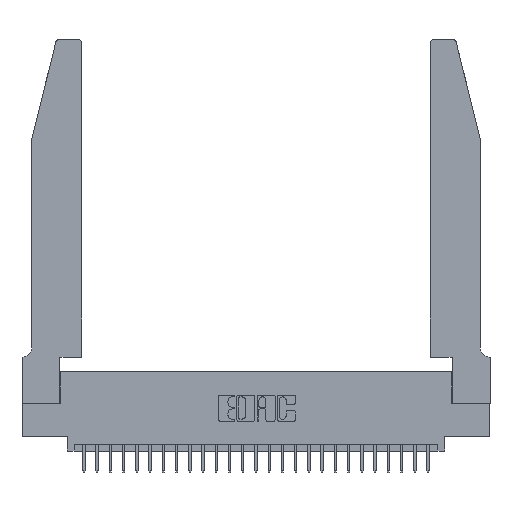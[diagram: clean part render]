
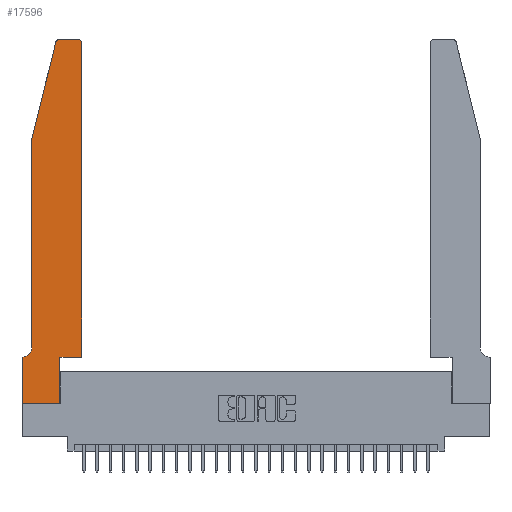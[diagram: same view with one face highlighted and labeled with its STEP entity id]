
A CAD part, top view. The second image highlights one B-rep face of the part: STEP entity #17596.
In plain terms, the highlighted planar face has unit normal (0, 0, 1).
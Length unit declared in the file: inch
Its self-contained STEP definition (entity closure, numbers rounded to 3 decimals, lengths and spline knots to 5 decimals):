
#159 = CARTESIAN_POINT ( 'NONE',  ( 0.284, 2.72, 0.37 ) ) ;
#443 = PLANE ( 'NONE',  #22139 ) ;
#631 = CARTESIAN_POINT ( 'NONE',  ( 0.2865, 0., 0.37 ) ) ;
#815 = DIRECTION ( 'NONE',  ( -1., 0., 0. ) ) ;
#893 = ORIENTED_EDGE ( 'NONE', *, *, #7026, .T. ) ;
#1359 = LINE ( 'NONE', #11806, #23803 ) ;
#1435 = VERTEX_POINT ( 'NONE', #25277 ) ;
#1686 = ORIENTED_EDGE ( 'NONE', *, *, #3947, .T. ) ;
#1898 = CIRCLE ( 'NONE', #14327, 0.07 ) ;
#2181 = DIRECTION ( 'NONE',  ( -1., 0., 0. ) ) ;
#2206 = CARTESIAN_POINT ( 'NONE',  ( 0.4505, 0.35, 0.37 ) ) ;
#2349 = CARTESIAN_POINT ( 'NONE',  ( 0.0755, 2., 0.37 ) ) ;
#2489 = DIRECTION ( 'NONE',  ( 1., 0., 0. ) ) ;
#3582 = CARTESIAN_POINT ( 'NONE',  ( 0., 0., 0.37 ) ) ;
#3947 = EDGE_CURVE ( 'NONE', #19488, #25809, #1359, .T. ) ;
#4549 = VECTOR ( 'NONE', #9200, 39.37008 ) ;
#4614 = DIRECTION ( 'NONE',  ( 0., -1., 0. ) ) ;
#4648 = EDGE_CURVE ( 'NONE', #10174, #25925, #24745, .T. ) ;
#4990 = DIRECTION ( 'NONE',  ( 0., 0., 1. ) ) ;
#5090 = DIRECTION ( 'NONE',  ( 0., 0., 1. ) ) ;
#5293 = ORIENTED_EDGE ( 'NONE', *, *, #12631, .T. ) ;
#5517 = AXIS2_PLACEMENT_3D ( 'NONE', #159, #15505, #2489 ) ;
#5609 = VERTEX_POINT ( 'NONE', #19052 ) ;
#6517 = ORIENTED_EDGE ( 'NONE', *, *, #21836, .T. ) ;
#7026 = EDGE_CURVE ( 'NONE', #5609, #13934, #12187, .T. ) ;
#7449 = VECTOR ( 'NONE', #4614, 39.37008 ) ;
#7740 = ORIENTED_EDGE ( 'NONE', *, *, #13269, .T. ) ;
#7753 = EDGE_CURVE ( 'NONE', #24947, #1435, #21922, .T. ) ;
#8119 = CARTESIAN_POINT ( 'NONE',  ( 0.2865, 0.35, 0.37 ) ) ;
#8923 = CARTESIAN_POINT ( 'NONE',  ( 0.0755, 2., 0.37 ) ) ;
#9200 = DIRECTION ( 'NONE',  ( 0., 1., 0. ) ) ;
#9277 = EDGE_CURVE ( 'NONE', #13934, #20509, #24633, .T. ) ;
#9488 = AXIS2_PLACEMENT_3D ( 'NONE', #18006, #5090, #20184 ) ;
#9513 = ORIENTED_EDGE ( 'NONE', *, *, #4648, .T. ) ;
#9641 = DIRECTION ( 'NONE',  ( 1., 0., 0. ) ) ;
#10174 = VERTEX_POINT ( 'NONE', #16843 ) ;
#11126 = VECTOR ( 'NONE', #9641, 39.37008 ) ;
#11675 = ORIENTED_EDGE ( 'NONE', *, *, #7753, .T. ) ;
#11806 = CARTESIAN_POINT ( 'NONE',  ( 0.2605, 2.75, 0.37 ) ) ;
#12187 = LINE ( 'NONE', #8923, #17905 ) ;
#12242 = CARTESIAN_POINT ( 'NONE',  ( 0., 0., 0.37 ) ) ;
#12516 = CARTESIAN_POINT ( 'NONE',  ( 0.4205, 2.75, 0.37 ) ) ;
#12631 = EDGE_CURVE ( 'NONE', #1435, #17283, #25854, .T. ) ;
#12876 = CIRCLE ( 'NONE', #5517, 0.03 ) ;
#13269 = EDGE_CURVE ( 'NONE', #26946, #24947, #21765, .T. ) ;
#13934 = VERTEX_POINT ( 'NONE', #25986 ) ;
#14024 = CARTESIAN_POINT ( 'NONE',  ( 0.0755, 0.35, 0.37 ) ) ;
#14327 = AXIS2_PLACEMENT_3D ( 'NONE', #28095, #15198, #2181 ) ;
#14463 = ORIENTED_EDGE ( 'NONE', *, *, #26116, .T. ) ;
#15198 = DIRECTION ( 'NONE',  ( 0., 0., -1. ) ) ;
#15223 = DIRECTION ( 'NONE',  ( 0., 1., 0. ) ) ;
#15376 = LINE ( 'NONE', #3582, #26164 ) ;
#15505 = DIRECTION ( 'NONE',  ( 0., 0., 1. ) ) ;
#15629 = FACE_OUTER_BOUND ( 'NONE', #18023, .T. ) ;
#15644 = EDGE_CURVE ( 'NONE', #25368, #10174, #16778, .T. ) ;
#16150 = DIRECTION ( 'NONE',  ( -1., 0., 0. ) ) ;
#16542 = DIRECTION ( 'NONE',  ( 1., 0., 0. ) ) ;
#16617 = CARTESIAN_POINT ( 'NONE',  ( 0., 0., 0.37 ) ) ;
#16778 = LINE ( 'NONE', #14024, #21154 ) ;
#16843 = CARTESIAN_POINT ( 'NONE',  ( 0., 0.35, 0.37 ) ) ;
#16967 = ORIENTED_EDGE ( 'NONE', *, *, #18683, .T. ) ;
#17283 = VERTEX_POINT ( 'NONE', #25377 ) ;
#17596 = ADVANCED_FACE ( 'NONE', ( #15629 ), #443, .T. ) ;
#17847 = ORIENTED_EDGE ( 'NONE', *, *, #26317, .T. ) ;
#17905 = VECTOR ( 'NONE', #23905, 39.37008 ) ;
#17909 = CARTESIAN_POINT ( 'NONE',  ( 0., 0.35, 0.37 ) ) ;
#18006 = CARTESIAN_POINT ( 'NONE',  ( 0.4205, 2.72, 0.37 ) ) ;
#18023 = EDGE_LOOP ( 'NONE', ( #1686, #16967, #893, #25917, #14463, #20744, #9513, #6517, #7740, #11675, #5293, #17847 ) ) ;
#18494 = CARTESIAN_POINT ( 'NONE',  ( 0.284, 2.75, 0.37 ) ) ;
#18683 = EDGE_CURVE ( 'NONE', #25809, #5609, #12876, .T. ) ;
#18850 = CARTESIAN_POINT ( 'NONE',  ( 0.0755, 0.42, 0.37 ) ) ;
#19009 = VECTOR ( 'NONE', #25138, 39.37008 ) ;
#19052 = CARTESIAN_POINT ( 'NONE',  ( 0.25487, 2.72718, 0.37 ) ) ;
#19488 = VERTEX_POINT ( 'NONE', #12516 ) ;
#19539 = CIRCLE ( 'NONE', #9488, 0.03 ) ;
#20086 = DIRECTION ( 'NONE',  ( 1., 0., 0. ) ) ;
#20184 = DIRECTION ( 'NONE',  ( 1., 0., 0. ) ) ;
#20509 = VERTEX_POINT ( 'NONE', #18850 ) ;
#20744 = ORIENTED_EDGE ( 'NONE', *, *, #15644, .T. ) ;
#21154 = VECTOR ( 'NONE', #815, 39.37008 ) ;
#21765 = LINE ( 'NONE', #24236, #4549 ) ;
#21836 = EDGE_CURVE ( 'NONE', #25925, #26946, #15376, .T. ) ;
#21922 = LINE ( 'NONE', #24687, #11126 ) ;
#22139 = AXIS2_PLACEMENT_3D ( 'NONE', #17909, #4990, #20086 ) ;
#23803 = VECTOR ( 'NONE', #16150, 39.37008 ) ;
#23905 = DIRECTION ( 'NONE',  ( -0.239, -0.971, 0. ) ) ;
#24236 = CARTESIAN_POINT ( 'NONE',  ( 0.2865, 0.35, 0.37 ) ) ;
#24633 = LINE ( 'NONE', #2349, #7449 ) ;
#24687 = CARTESIAN_POINT ( 'NONE',  ( 0.4505, 0.35, 0.37 ) ) ;
#24745 = LINE ( 'NONE', #12242, #19009 ) ;
#24947 = VERTEX_POINT ( 'NONE', #8119 ) ;
#25138 = DIRECTION ( 'NONE',  ( 0., -1., 0. ) ) ;
#25149 = VECTOR ( 'NONE', #15223, 39.37008 ) ;
#25277 = CARTESIAN_POINT ( 'NONE',  ( 0.4505, 0.35, 0.37 ) ) ;
#25368 = VERTEX_POINT ( 'NONE', #25613 ) ;
#25377 = CARTESIAN_POINT ( 'NONE',  ( 0.4505, 2.72, 0.37 ) ) ;
#25613 = CARTESIAN_POINT ( 'NONE',  ( 0.0055, 0.35, 0.37 ) ) ;
#25809 = VERTEX_POINT ( 'NONE', #18494 ) ;
#25854 = LINE ( 'NONE', #2206, #25149 ) ;
#25917 = ORIENTED_EDGE ( 'NONE', *, *, #9277, .T. ) ;
#25925 = VERTEX_POINT ( 'NONE', #16617 ) ;
#25986 = CARTESIAN_POINT ( 'NONE',  ( 0.0755, 2., 0.37 ) ) ;
#26116 = EDGE_CURVE ( 'NONE', #20509, #25368, #1898, .T. ) ;
#26164 = VECTOR ( 'NONE', #16542, 39.37008 ) ;
#26317 = EDGE_CURVE ( 'NONE', #17283, #19488, #19539, .T. ) ;
#26946 = VERTEX_POINT ( 'NONE', #631 ) ;
#28095 = CARTESIAN_POINT ( 'NONE',  ( 0.0055, 0.42, 0.37 ) ) ;
